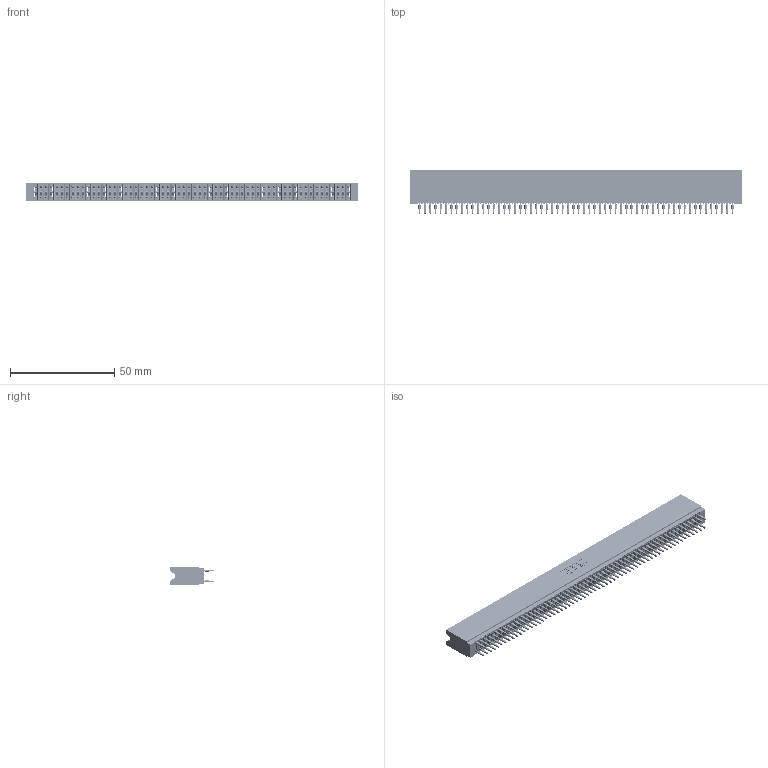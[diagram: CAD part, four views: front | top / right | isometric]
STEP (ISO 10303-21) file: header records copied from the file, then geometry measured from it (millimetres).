
FILE_DESCRIPTION (( 'STEP AP203' ), '1' );
FILE_NAME ('745-120-560-206.STEP', '2020-09-14T17:16:46', ( '' ), ( '' ), 'SwSTEP 2.0', 'SolidWorks 2020', '' );
FILE_SCHEMA (( 'CONFIG_CONTROL_DESIGN' ));
Products named in the file (3): 745-292-001_560; 745-120-560-206; 745 Part_Insulator Option - 06
Assembly tree (121 placements, depth 2):
  745-120-560-206
    745 Part_Insulator Option - 06
    745-292-001_560  x120
Bounding box: 159 x 21.22 x 8.89 mm (x, y, z)
Volume: 14632 mm3; surface area: 32082.7 mm2
Topology: 121 solids, 121 shells, 11916 faces, 32600 edges, 20692 vertices
Faces by surface type: plane 6176, cylinder 2620, bspline 2400, torus 720
Entity records: 98903 total; most frequent: CARTESIAN_POINT 17652, ORIENTED_EDGE 17124, DIRECTION 14948, EDGE_CURVE 8562, LINE 8012, VECTOR 8012, VERTEX_POINT 5460, AXIS2_PLACEMENT_3D 3468
